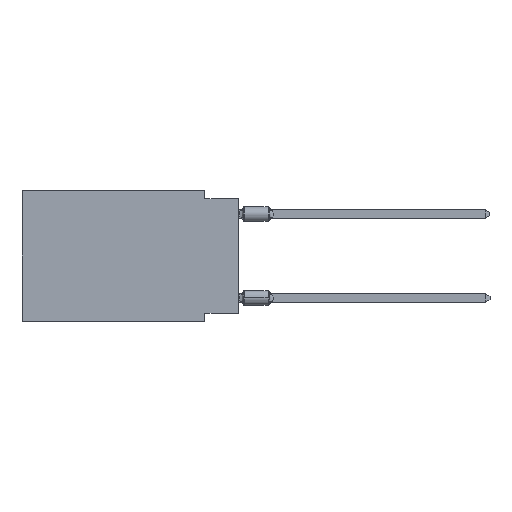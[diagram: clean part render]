
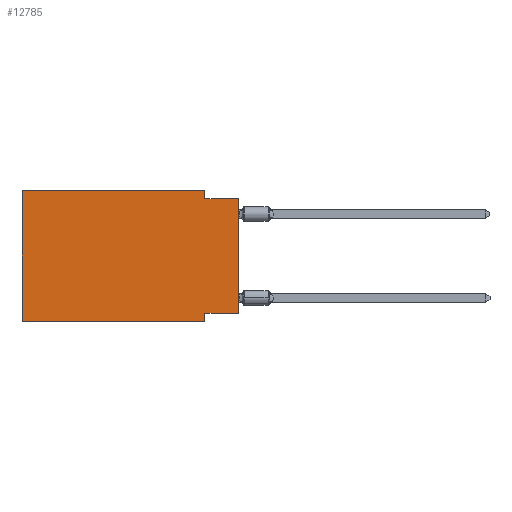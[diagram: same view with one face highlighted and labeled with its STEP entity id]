
A CAD part, left-side view. The second image highlights one B-rep face of the part: STEP entity #12785.
In plain terms, the highlighted planar face has unit normal (-1, 0, 0).
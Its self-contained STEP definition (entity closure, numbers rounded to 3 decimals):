
#341 = CARTESIAN_POINT ( 'NONE',  ( 0., 2.54, -9.906 ) ) ;
#533 = EDGE_CURVE ( 'NONE', #12811, #27239, #16437, .T. ) ;
#737 = CARTESIAN_POINT ( 'NONE',  ( 0., 16.383, -9.906 ) ) ;
#778 = EDGE_CURVE ( 'NONE', #24847, #15437, #10768, .T. ) ;
#1289 = DIRECTION ( 'NONE',  ( 0., 0., -1. ) ) ;
#1535 = CARTESIAN_POINT ( 'NONE',  ( 0., 0., -0.635 ) ) ;
#2135 = VECTOR ( 'NONE', #10238, 1000. ) ;
#3269 = DIRECTION ( 'NONE',  ( 1., 0., 0. ) ) ;
#3378 = VECTOR ( 'NONE', #28321, 1000. ) ;
#3752 = CARTESIAN_POINT ( 'NONE',  ( 0., 0., -9.271 ) ) ;
#3796 = EDGE_CURVE ( 'NONE', #12811, #24847, #19867, .T. ) ;
#4673 = ORIENTED_EDGE ( 'NONE', *, *, #778, .F. ) ;
#5430 = LINE ( 'NONE', #12222, #21358 ) ;
#6091 = FACE_OUTER_BOUND ( 'NONE', #15813, .T. ) ;
#6239 = ORIENTED_EDGE ( 'NONE', *, *, #533, .T. ) ;
#7665 = EDGE_CURVE ( 'NONE', #18627, #27239, #20986, .T. ) ;
#8128 = CARTESIAN_POINT ( 'NONE',  ( 0., 0., -0.635 ) ) ;
#8352 = PLANE ( 'NONE',  #19346 ) ;
#8388 = DIRECTION ( 'NONE',  ( 0., 0., 1. ) ) ;
#10238 = DIRECTION ( 'NONE',  ( 0., -1., 0. ) ) ;
#10262 = ORIENTED_EDGE ( 'NONE', *, *, #29143, .T. ) ;
#10623 = DIRECTION ( 'NONE',  ( 0., -1., 0. ) ) ;
#10708 = CARTESIAN_POINT ( 'NONE',  ( 0., 2.54, 0. ) ) ;
#10768 = LINE ( 'NONE', #19286, #18598 ) ;
#10939 = VECTOR ( 'NONE', #8388, 1000. ) ;
#12222 = CARTESIAN_POINT ( 'NONE',  ( 0., 0., 0. ) ) ;
#12261 = LINE ( 'NONE', #27101, #22894 ) ;
#12785 = ADVANCED_FACE ( 'NONE', ( #6091 ), #8352, .F. ) ;
#12811 = VERTEX_POINT ( 'NONE', #26308 ) ;
#13075 = EDGE_CURVE ( 'NONE', #15437, #18893, #12261, .T. ) ;
#13424 = LINE ( 'NONE', #18115, #29681 ) ;
#15306 = CARTESIAN_POINT ( 'NONE',  ( 0., 16.383, 0. ) ) ;
#15437 = VERTEX_POINT ( 'NONE', #10708 ) ;
#15813 = EDGE_LOOP ( 'NONE', ( #10262, #24597, #19345, #4673, #23265, #6239, #21361, #21386 ) ) ;
#16437 = LINE ( 'NONE', #737, #3378 ) ;
#17026 = CARTESIAN_POINT ( 'NONE',  ( 0., 16.383, 0. ) ) ;
#18115 = CARTESIAN_POINT ( 'NONE',  ( 0., 0., -9.271 ) ) ;
#18598 = VECTOR ( 'NONE', #10623, 1000. ) ;
#18627 = VERTEX_POINT ( 'NONE', #22837 ) ;
#18893 = VERTEX_POINT ( 'NONE', #28917 ) ;
#19286 = CARTESIAN_POINT ( 'NONE',  ( 0., 16.383, 0. ) ) ;
#19345 = ORIENTED_EDGE ( 'NONE', *, *, #13075, .F. ) ;
#19346 = AXIS2_PLACEMENT_3D ( 'NONE', #15306, #3269, #1289 ) ;
#19620 = EDGE_CURVE ( 'NONE', #25844, #18627, #13424, .T. ) ;
#19867 = LINE ( 'NONE', #17026, #10939 ) ;
#20986 = LINE ( 'NONE', #341, #23693 ) ;
#21358 = VECTOR ( 'NONE', #24271, 1000. ) ;
#21361 = ORIENTED_EDGE ( 'NONE', *, *, #7665, .F. ) ;
#21386 = ORIENTED_EDGE ( 'NONE', *, *, #19620, .F. ) ;
#22467 = DIRECTION ( 'NONE',  ( 0., 0., -1. ) ) ;
#22813 = CARTESIAN_POINT ( 'NONE',  ( 0., 2.54, -9.906 ) ) ;
#22837 = CARTESIAN_POINT ( 'NONE',  ( 0., 2.54, -9.271 ) ) ;
#22894 = VECTOR ( 'NONE', #22467, 1000. ) ;
#23265 = ORIENTED_EDGE ( 'NONE', *, *, #3796, .F. ) ;
#23396 = DIRECTION ( 'NONE',  ( 0., 0., -1. ) ) ;
#23693 = VECTOR ( 'NONE', #23396, 1000. ) ;
#24271 = DIRECTION ( 'NONE',  ( 0., 0., 1. ) ) ;
#24597 = ORIENTED_EDGE ( 'NONE', *, *, #27792, .F. ) ;
#24847 = VERTEX_POINT ( 'NONE', #28297 ) ;
#25172 = DIRECTION ( 'NONE',  ( 0., 1., 0. ) ) ;
#25844 = VERTEX_POINT ( 'NONE', #3752 ) ;
#26308 = CARTESIAN_POINT ( 'NONE',  ( 0., 16.383, -9.906 ) ) ;
#27101 = CARTESIAN_POINT ( 'NONE',  ( 0., 2.54, 0. ) ) ;
#27239 = VERTEX_POINT ( 'NONE', #22813 ) ;
#27621 = VERTEX_POINT ( 'NONE', #1535 ) ;
#27792 = EDGE_CURVE ( 'NONE', #18893, #27621, #27901, .T. ) ;
#27901 = LINE ( 'NONE', #8128, #2135 ) ;
#28297 = CARTESIAN_POINT ( 'NONE',  ( 0., 16.383, 0. ) ) ;
#28321 = DIRECTION ( 'NONE',  ( 0., -1., 0. ) ) ;
#28917 = CARTESIAN_POINT ( 'NONE',  ( 0., 2.54, -0.635 ) ) ;
#29143 = EDGE_CURVE ( 'NONE', #25844, #27621, #5430, .T. ) ;
#29681 = VECTOR ( 'NONE', #25172, 1000. ) ;
